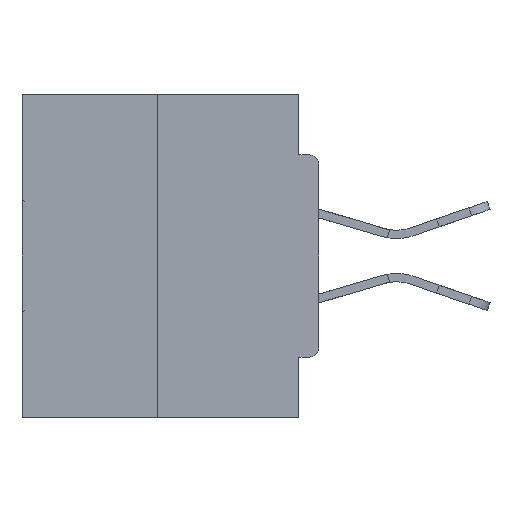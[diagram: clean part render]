
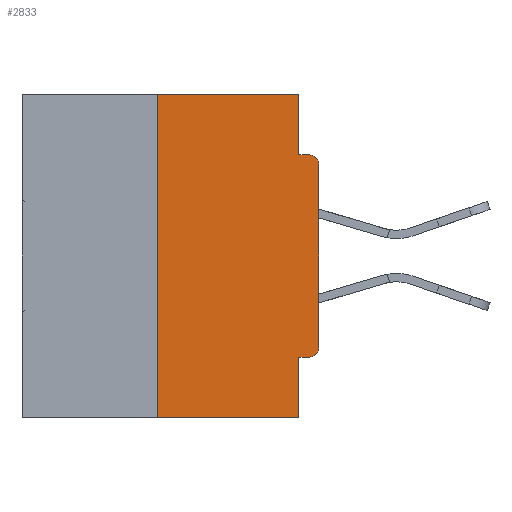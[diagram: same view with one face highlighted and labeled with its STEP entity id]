
A CAD part, left-side view. The second image highlights one B-rep face of the part: STEP entity #2833.
In plain terms, the highlighted planar face has unit normal (-1, 0, 0).
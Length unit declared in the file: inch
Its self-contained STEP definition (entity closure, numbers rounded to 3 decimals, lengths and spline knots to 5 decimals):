
#262 = EDGE_LOOP ( 'NONE', ( #21265, #2650, #32882, #15884, #38055, #22509, #9225, #28293, #38451, #35379 ) ) ;
#311 = CARTESIAN_POINT ( 'NONE',  ( 0., 0.031, -0.0935 ) ) ;
#373 = EDGE_CURVE ( 'NONE', #28310, #5520, #4065, .T. ) ;
#583 = VECTOR ( 'NONE', #1548, 39.37008 ) ;
#685 = AXIS2_PLACEMENT_3D ( 'NONE', #12542, #22406, #20507 ) ;
#1197 = VECTOR ( 'NONE', #30392, 39.37008 ) ;
#1548 = DIRECTION ( 'NONE',  ( 0., 0., -1. ) ) ;
#1851 = CARTESIAN_POINT ( 'NONE',  ( 0., 0.031, -0.5 ) ) ;
#2641 = CARTESIAN_POINT ( 'NONE',  ( 0., 0.015, -0.4065 ) ) ;
#2650 = ORIENTED_EDGE ( 'NONE', *, *, #7435, .F. ) ;
#2833 = ADVANCED_FACE ( 'NONE', ( #40736 ), #21031, .F. ) ;
#3154 = EDGE_CURVE ( 'NONE', #21221, #32722, #29428, .T. ) ;
#4065 = LINE ( 'NONE', #36054, #20440 ) ;
#4197 = VERTEX_POINT ( 'NONE', #27096 ) ;
#4256 = VECTOR ( 'NONE', #35978, 39.37008 ) ;
#4916 = CARTESIAN_POINT ( 'NONE',  ( 0., 0.031, -0.5 ) ) ;
#5520 = VERTEX_POINT ( 'NONE', #4916 ) ;
#6306 = LINE ( 'NONE', #35970, #1197 ) ;
#6769 = VECTOR ( 'NONE', #15033, 39.37008 ) ;
#7112 = CIRCLE ( 'NONE', #685, 0.015 ) ;
#7435 = EDGE_CURVE ( 'NONE', #28310, #14277, #6306, .T. ) ;
#8070 = EDGE_CURVE ( 'NONE', #4197, #5520, #12927, .T. ) ;
#8129 = EDGE_CURVE ( 'NONE', #42074, #32807, #14973, .T. ) ;
#8789 = VECTOR ( 'NONE', #19066, 39.37008 ) ;
#8877 = LINE ( 'NONE', #16753, #4256 ) ;
#9225 = ORIENTED_EDGE ( 'NONE', *, *, #15329, .T. ) ;
#9473 = CARTESIAN_POINT ( 'NONE',  ( 0., 0., -0.0935 ) ) ;
#10299 = VECTOR ( 'NONE', #40643, 39.37008 ) ;
#10815 = LINE ( 'NONE', #9473, #8789 ) ;
#11215 = CARTESIAN_POINT ( 'NONE',  ( 0., 0., -0.1085 ) ) ;
#11468 = DIRECTION ( 'NONE',  ( 0., -1., 0. ) ) ;
#12542 = CARTESIAN_POINT ( 'NONE',  ( 0., 0.015, -0.3915 ) ) ;
#12927 = LINE ( 'NONE', #1851, #6769 ) ;
#14277 = VERTEX_POINT ( 'NONE', #18112 ) ;
#14310 = CARTESIAN_POINT ( 'NONE',  ( 0., 0.46, 0. ) ) ;
#14973 = LINE ( 'NONE', #24333, #583 ) ;
#15033 = DIRECTION ( 'NONE',  ( 0., 0., -1. ) ) ;
#15329 = EDGE_CURVE ( 'NONE', #41904, #21221, #8877, .T. ) ;
#15884 = ORIENTED_EDGE ( 'NONE', *, *, #8070, .F. ) ;
#16001 = CARTESIAN_POINT ( 'NONE',  ( 0., 0.015, -0.1085 ) ) ;
#16594 = EDGE_CURVE ( 'NONE', #14277, #42074, #22573, .T. ) ;
#16753 = CARTESIAN_POINT ( 'NONE',  ( 0., 0., 0. ) ) ;
#17251 = CARTESIAN_POINT ( 'NONE',  ( 0., 0., -0.4065 ) ) ;
#17667 = CARTESIAN_POINT ( 'NONE',  ( 0., 0.25, -0.5 ) ) ;
#18112 = CARTESIAN_POINT ( 'NONE',  ( 0., 0.25, 0. ) ) ;
#19066 = DIRECTION ( 'NONE',  ( 0., -1., 0. ) ) ;
#19696 = AXIS2_PLACEMENT_3D ( 'NONE', #16001, #30664, #26052 ) ;
#20440 = VECTOR ( 'NONE', #25909, 39.37008 ) ;
#20507 = DIRECTION ( 'NONE',  ( 0., 0., -1. ) ) ;
#20520 = VECTOR ( 'NONE', #11468, 39.37008 ) ;
#21031 = PLANE ( 'NONE',  #23533 ) ;
#21221 = VERTEX_POINT ( 'NONE', #11215 ) ;
#21265 = ORIENTED_EDGE ( 'NONE', *, *, #16594, .F. ) ;
#22406 = DIRECTION ( 'NONE',  ( -1., 0., 0. ) ) ;
#22509 = ORIENTED_EDGE ( 'NONE', *, *, #33693, .T. ) ;
#22573 = LINE ( 'NONE', #34797, #20520 ) ;
#23533 = AXIS2_PLACEMENT_3D ( 'NONE', #14310, #23915, #27226 ) ;
#23915 = DIRECTION ( 'NONE',  ( 1., 0., 0. ) ) ;
#24333 = CARTESIAN_POINT ( 'NONE',  ( 0., 0.031, 0. ) ) ;
#24693 = EDGE_CURVE ( 'NONE', #26878, #4197, #27760, .T. ) ;
#25909 = DIRECTION ( 'NONE',  ( 0., -1., 0. ) ) ;
#26052 = DIRECTION ( 'NONE',  ( 0., 0., -1. ) ) ;
#26878 = VERTEX_POINT ( 'NONE', #2641 ) ;
#27096 = CARTESIAN_POINT ( 'NONE',  ( 0., 0.031, -0.4065 ) ) ;
#27226 = DIRECTION ( 'NONE',  ( 0., 0., -1. ) ) ;
#27760 = LINE ( 'NONE', #17251, #10299 ) ;
#28293 = ORIENTED_EDGE ( 'NONE', *, *, #3154, .T. ) ;
#28310 = VERTEX_POINT ( 'NONE', #17667 ) ;
#29428 = CIRCLE ( 'NONE', #19696, 0.015 ) ;
#30392 = DIRECTION ( 'NONE',  ( 0., 0., 1. ) ) ;
#30664 = DIRECTION ( 'NONE',  ( -1., 0., 0. ) ) ;
#31660 = EDGE_CURVE ( 'NONE', #32807, #32722, #10815, .T. ) ;
#32722 = VERTEX_POINT ( 'NONE', #41754 ) ;
#32807 = VERTEX_POINT ( 'NONE', #311 ) ;
#32882 = ORIENTED_EDGE ( 'NONE', *, *, #373, .T. ) ;
#33693 = EDGE_CURVE ( 'NONE', #26878, #41904, #7112, .T. ) ;
#34797 = CARTESIAN_POINT ( 'NONE',  ( 0., 0.46, 0. ) ) ;
#35379 = ORIENTED_EDGE ( 'NONE', *, *, #8129, .F. ) ;
#35970 = CARTESIAN_POINT ( 'NONE',  ( 0., 0.25, 0. ) ) ;
#35978 = DIRECTION ( 'NONE',  ( 0., 0., 1. ) ) ;
#36054 = CARTESIAN_POINT ( 'NONE',  ( 0., 0.46, -0.5 ) ) ;
#38055 = ORIENTED_EDGE ( 'NONE', *, *, #24693, .F. ) ;
#38451 = ORIENTED_EDGE ( 'NONE', *, *, #31660, .F. ) ;
#40221 = CARTESIAN_POINT ( 'NONE',  ( 0., 0.031, 0. ) ) ;
#40643 = DIRECTION ( 'NONE',  ( 0., 1., 0. ) ) ;
#40736 = FACE_OUTER_BOUND ( 'NONE', #262, .T. ) ;
#41754 = CARTESIAN_POINT ( 'NONE',  ( 0., 0.015, -0.0935 ) ) ;
#41904 = VERTEX_POINT ( 'NONE', #42155 ) ;
#42074 = VERTEX_POINT ( 'NONE', #40221 ) ;
#42155 = CARTESIAN_POINT ( 'NONE',  ( 0., 0., -0.3915 ) ) ;
